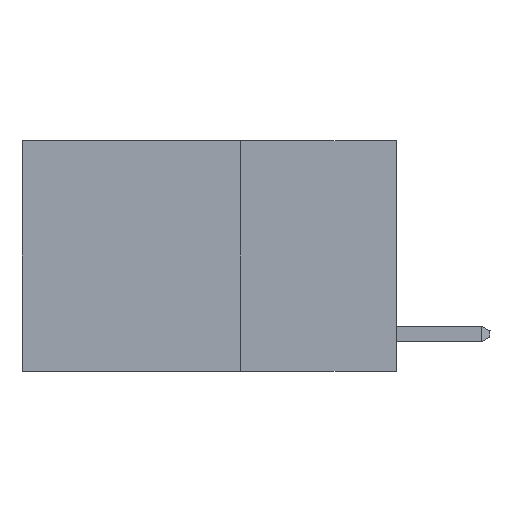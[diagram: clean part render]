
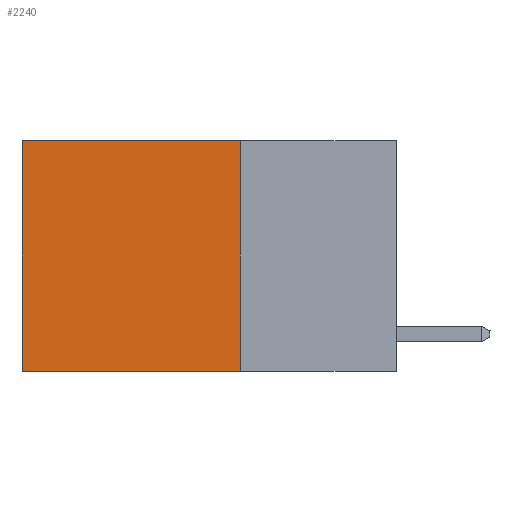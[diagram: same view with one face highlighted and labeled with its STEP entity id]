
A CAD part, left-side view. The second image highlights one B-rep face of the part: STEP entity #2240.
In plain terms, the highlighted planar face has unit normal (-1, 0, 0).
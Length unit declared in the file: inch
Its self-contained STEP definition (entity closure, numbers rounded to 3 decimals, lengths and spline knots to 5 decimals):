
#164 = EDGE_LOOP ( 'NONE', ( #6399, #18860, #17220, #882 ) ) ;
#335 = DIRECTION ( 'NONE',  ( 0., 0., -1. ) ) ;
#882 = ORIENTED_EDGE ( 'NONE', *, *, #3715, .T. ) ;
#1316 = VECTOR ( 'NONE', #8706, 39.37008 ) ;
#2065 = CARTESIAN_POINT ( 'NONE',  ( 0.2625, 0.25, 0. ) ) ;
#2151 = CARTESIAN_POINT ( 'NONE',  ( 0.2625, 0.25, 0. ) ) ;
#2240 = ADVANCED_FACE ( 'NONE', ( #20768 ), #7072, .F. ) ;
#2396 = EDGE_CURVE ( 'NONE', #15644, #13215, #7472, .T. ) ;
#3715 = EDGE_CURVE ( 'NONE', #11396, #3823, #19284, .T. ) ;
#3823 = VERTEX_POINT ( 'NONE', #5538 ) ;
#4200 = EDGE_CURVE ( 'NONE', #11396, #15644, #14734, .T. ) ;
#4933 = CARTESIAN_POINT ( 'NONE',  ( 0.2625, 0.25, -0.37 ) ) ;
#5538 = CARTESIAN_POINT ( 'NONE',  ( 0.2625, 0.6, 0. ) ) ;
#5657 = CARTESIAN_POINT ( 'NONE',  ( 0.2625, 0.6, -0.37 ) ) ;
#5690 = DIRECTION ( 'NONE',  ( 0., 0., -1. ) ) ;
#5921 = DIRECTION ( 'NONE',  ( 0., 0., -1. ) ) ;
#6010 = VECTOR ( 'NONE', #5921, 39.37008 ) ;
#6399 = ORIENTED_EDGE ( 'NONE', *, *, #16323, .T. ) ;
#7072 = PLANE ( 'NONE',  #8376 ) ;
#7472 = LINE ( 'NONE', #10341, #10014 ) ;
#7564 = CARTESIAN_POINT ( 'NONE',  ( 0.2625, 0.25, 0. ) ) ;
#8376 = AXIS2_PLACEMENT_3D ( 'NONE', #2151, #13713, #335 ) ;
#8706 = DIRECTION ( 'NONE',  ( 0., 1., 0. ) ) ;
#10014 = VECTOR ( 'NONE', #17334, 39.37008 ) ;
#10341 = CARTESIAN_POINT ( 'NONE',  ( 0.2625, 0.25, -0.37 ) ) ;
#11396 = VERTEX_POINT ( 'NONE', #2065 ) ;
#11902 = LINE ( 'NONE', #18227, #18059 ) ;
#13215 = VERTEX_POINT ( 'NONE', #5657 ) ;
#13713 = DIRECTION ( 'NONE',  ( 1., 0., 0. ) ) ;
#14734 = LINE ( 'NONE', #7564, #6010 ) ;
#15314 = CARTESIAN_POINT ( 'NONE',  ( 0.2625, 0.25, 0. ) ) ;
#15644 = VERTEX_POINT ( 'NONE', #4933 ) ;
#16323 = EDGE_CURVE ( 'NONE', #3823, #13215, #11902, .T. ) ;
#17220 = ORIENTED_EDGE ( 'NONE', *, *, #4200, .F. ) ;
#17334 = DIRECTION ( 'NONE',  ( 0., 1., 0. ) ) ;
#18059 = VECTOR ( 'NONE', #5690, 39.37008 ) ;
#18227 = CARTESIAN_POINT ( 'NONE',  ( 0.2625, 0.6, 0. ) ) ;
#18860 = ORIENTED_EDGE ( 'NONE', *, *, #2396, .F. ) ;
#19284 = LINE ( 'NONE', #15314, #1316 ) ;
#20768 = FACE_OUTER_BOUND ( 'NONE', #164, .T. ) ;
